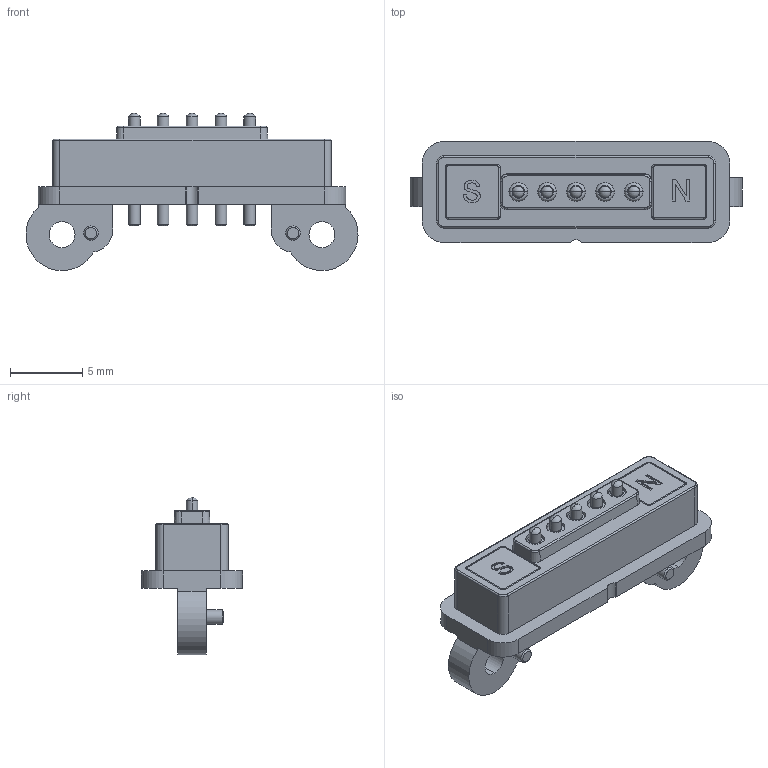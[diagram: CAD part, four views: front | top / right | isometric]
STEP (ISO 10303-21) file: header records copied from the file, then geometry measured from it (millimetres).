
FILE_DESCRIPTION (( 'STEP AP214' ), '1' );
FILE_NAME ('685J0521251114E.STEP', '2023-04-13T19:30:23', ( '' ), ( '' ), 'SwSTEP 2.0', 'SolidWorks 2020', '' );
FILE_SCHEMA (( 'AUTOMOTIVE_DESIGN' ));
Length unit declared in the file: millimetre
Products named in the file (1): 685J0521251114E
Bounding box: 23 x 7 x 10.9 mm (x, y, z)
Volume: 554.3 mm3; surface area: 947 mm2
Topology: 6 solids, 13 shells, 330 faces, 742 edges, 458 vertices
Faces by surface type: cylinder 135, plane 104, cone 33, bspline 26, torus 22, sphere 10
Entity records: 13873 total; most frequent: CARTESIAN_POINT 2627, DIRECTION 1672, ORIENTED_EDGE 1484, EDGE_CURVE 742, AXIS2_PLACEMENT_3D 655, VERTEX_POINT 458, EDGE_LOOP 368, LINE 362
